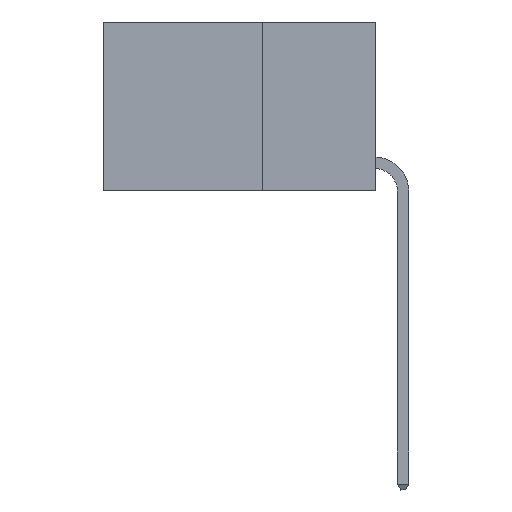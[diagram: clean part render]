
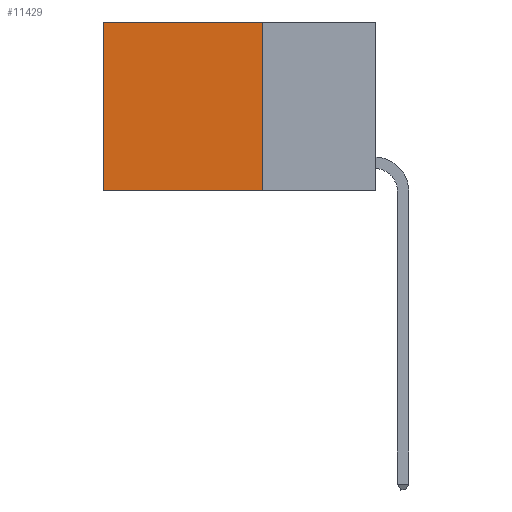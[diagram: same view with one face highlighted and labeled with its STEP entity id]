
A CAD part, left-side view. The second image highlights one B-rep face of the part: STEP entity #11429.
In plain terms, the highlighted planar face has unit normal (-1, 0, 0).
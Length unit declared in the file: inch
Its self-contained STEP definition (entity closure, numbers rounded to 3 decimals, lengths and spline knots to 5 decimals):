
#292 = AXIS2_PLACEMENT_3D ( 'NONE', #12313, #4555, #7614 ) ;
#677 = ORIENTED_EDGE ( 'NONE', *, *, #2945, .F. ) ;
#796 = VECTOR ( 'NONE', #6207, 39.37008 ) ;
#1100 = LINE ( 'NONE', #1158, #6734 ) ;
#1158 = CARTESIAN_POINT ( 'NONE',  ( 0.2625, 0.25, -0.37 ) ) ;
#1976 = LINE ( 'NONE', #4307, #796 ) ;
#2945 = EDGE_CURVE ( 'NONE', #4617, #5776, #1100, .T. ) ;
#3095 = EDGE_CURVE ( 'NONE', #11880, #5776, #9443, .T. ) ;
#3166 = CARTESIAN_POINT ( 'NONE',  ( 0.2625, 0.25, 0. ) ) ;
#3554 = DIRECTION ( 'NONE',  ( 0., 0., -1. ) ) ;
#4307 = CARTESIAN_POINT ( 'NONE',  ( 0.2625, 0.25, 0. ) ) ;
#4372 = VECTOR ( 'NONE', #3554, 39.37008 ) ;
#4555 = DIRECTION ( 'NONE',  ( 1., 0., 0. ) ) ;
#4617 = VERTEX_POINT ( 'NONE', #7033 ) ;
#4937 = CARTESIAN_POINT ( 'NONE',  ( 0.2625, 0.6, -0.37 ) ) ;
#5620 = PLANE ( 'NONE',  #292 ) ;
#5776 = VERTEX_POINT ( 'NONE', #4937 ) ;
#5870 = EDGE_CURVE ( 'NONE', #6650, #4617, #1976, .T. ) ;
#6033 = ORIENTED_EDGE ( 'NONE', *, *, #3095, .T. ) ;
#6120 = LINE ( 'NONE', #3166, #9798 ) ;
#6158 = DIRECTION ( 'NONE',  ( 0., 1., 0. ) ) ;
#6207 = DIRECTION ( 'NONE',  ( 0., 0., -1. ) ) ;
#6650 = VERTEX_POINT ( 'NONE', #12490 ) ;
#6734 = VECTOR ( 'NONE', #6158, 39.37008 ) ;
#7033 = CARTESIAN_POINT ( 'NONE',  ( 0.2625, 0.25, -0.37 ) ) ;
#7614 = DIRECTION ( 'NONE',  ( 0., 0., -1. ) ) ;
#7800 = ORIENTED_EDGE ( 'NONE', *, *, #10571, .T. ) ;
#8693 = FACE_OUTER_BOUND ( 'NONE', #10879, .T. ) ;
#9443 = LINE ( 'NONE', #12077, #4372 ) ;
#9798 = VECTOR ( 'NONE', #10009, 39.37008 ) ;
#10009 = DIRECTION ( 'NONE',  ( 0., 1., 0. ) ) ;
#10571 = EDGE_CURVE ( 'NONE', #6650, #11880, #6120, .T. ) ;
#10879 = EDGE_LOOP ( 'NONE', ( #6033, #677, #12225, #7800 ) ) ;
#11218 = CARTESIAN_POINT ( 'NONE',  ( 0.2625, 0.6, 0. ) ) ;
#11429 = ADVANCED_FACE ( 'NONE', ( #8693 ), #5620, .F. ) ;
#11880 = VERTEX_POINT ( 'NONE', #11218 ) ;
#12077 = CARTESIAN_POINT ( 'NONE',  ( 0.2625, 0.6, 0. ) ) ;
#12225 = ORIENTED_EDGE ( 'NONE', *, *, #5870, .F. ) ;
#12313 = CARTESIAN_POINT ( 'NONE',  ( 0.2625, 0.25, 0. ) ) ;
#12490 = CARTESIAN_POINT ( 'NONE',  ( 0.2625, 0.25, 0. ) ) ;
